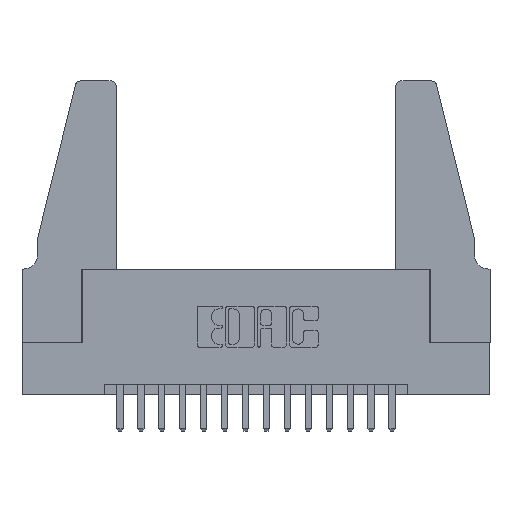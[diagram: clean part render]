
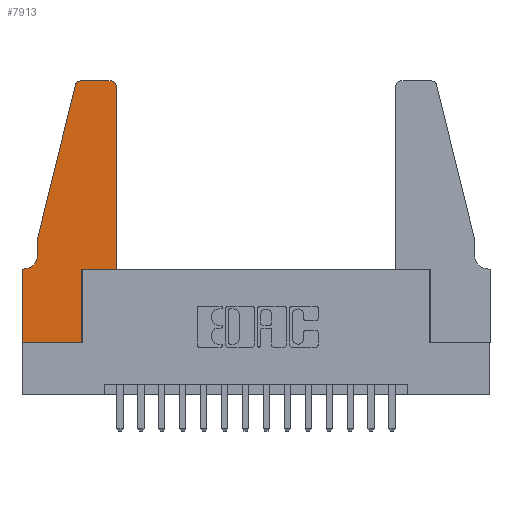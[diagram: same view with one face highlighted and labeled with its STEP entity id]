
A CAD part, top view. The second image highlights one B-rep face of the part: STEP entity #7913.
In plain terms, the highlighted planar face has unit normal (0, 0, 1).
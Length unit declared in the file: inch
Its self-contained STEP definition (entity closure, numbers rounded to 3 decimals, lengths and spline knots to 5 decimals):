
#458 = LINE ( 'NONE', #13785, #7588 ) ;
#483 = ORIENTED_EDGE ( 'NONE', *, *, #13686, .T. ) ;
#556 = CARTESIAN_POINT ( 'NONE',  ( 0., 0.35, 0.37 ) ) ;
#858 = EDGE_CURVE ( 'NONE', #5133, #15432, #12347, .T. ) ;
#1026 = DIRECTION ( 'NONE',  ( -0.239, -0.971, 0. ) ) ;
#1693 = VECTOR ( 'NONE', #9237, 39.37008 ) ;
#1851 = CARTESIAN_POINT ( 'NONE',  ( 0.4505, 1.22, 0.37 ) ) ;
#2402 = CARTESIAN_POINT ( 'NONE',  ( 0.4205, 1.25, 0.37 ) ) ;
#2616 = VECTOR ( 'NONE', #14030, 39.37008 ) ;
#3162 = EDGE_CURVE ( 'NONE', #16909, #5133, #6333, .T. ) ;
#3277 = DIRECTION ( 'NONE',  ( 1., 0., 0. ) ) ;
#3656 = VERTEX_POINT ( 'NONE', #10121 ) ;
#4007 = EDGE_LOOP ( 'NONE', ( #9129, #13714, #14220, #9911, #16022, #4185, #13271, #483, #8920, #12333, #10985, #10590 ) ) ;
#4185 = ORIENTED_EDGE ( 'NONE', *, *, #858, .T. ) ;
#4393 = EDGE_CURVE ( 'NONE', #14015, #13728, #16168, .T. ) ;
#4400 = VERTEX_POINT ( 'NONE', #2402 ) ;
#4958 = CARTESIAN_POINT ( 'NONE',  ( 0.0055, 0.42, 0.37 ) ) ;
#5133 = VERTEX_POINT ( 'NONE', #14228 ) ;
#5149 = CARTESIAN_POINT ( 'NONE',  ( 0.2865, 0., 0.37 ) ) ;
#5242 = LINE ( 'NONE', #13242, #12202 ) ;
#5379 = VECTOR ( 'NONE', #9715, 39.37008 ) ;
#5393 = DIRECTION ( 'NONE',  ( -1., 0., 0. ) ) ;
#5952 = DIRECTION ( 'NONE',  ( 0., 0., 1. ) ) ;
#6082 = CARTESIAN_POINT ( 'NONE',  ( 0.284, 1.25, 0.37 ) ) ;
#6154 = EDGE_CURVE ( 'NONE', #13728, #16909, #13134, .T. ) ;
#6277 = DIRECTION ( 'NONE',  ( -1., 0., 0. ) ) ;
#6333 = CIRCLE ( 'NONE', #15976, 0.07 ) ;
#6568 = CARTESIAN_POINT ( 'NONE',  ( 0.0755, 0.42, 0.37 ) ) ;
#6628 = CARTESIAN_POINT ( 'NONE',  ( 0.0755, 0.5, 0.37 ) ) ;
#6724 = CARTESIAN_POINT ( 'NONE',  ( 0.4505, 0.35, 0.37 ) ) ;
#7111 = DIRECTION ( 'NONE',  ( 0., 0., 1. ) ) ;
#7262 = DIRECTION ( 'NONE',  ( 1., 0., 0. ) ) ;
#7545 = CARTESIAN_POINT ( 'NONE',  ( 0.2865, 0.35, 0.37 ) ) ;
#7588 = VECTOR ( 'NONE', #7262, 39.37008 ) ;
#7666 = VERTEX_POINT ( 'NONE', #6724 ) ;
#7913 = ADVANCED_FACE ( 'NONE', ( #14283 ), #13766, .T. ) ;
#8058 = CIRCLE ( 'NONE', #16839, 0.03 ) ;
#8786 = EDGE_CURVE ( 'NONE', #7666, #14773, #10790, .T. ) ;
#8920 = ORIENTED_EDGE ( 'NONE', *, *, #12133, .T. ) ;
#9095 = AXIS2_PLACEMENT_3D ( 'NONE', #556, #11200, #3277 ) ;
#9129 = ORIENTED_EDGE ( 'NONE', *, *, #14505, .T. ) ;
#9237 = DIRECTION ( 'NONE',  ( 1., 0., 0. ) ) ;
#9715 = DIRECTION ( 'NONE',  ( -1., 0., 0. ) ) ;
#9911 = ORIENTED_EDGE ( 'NONE', *, *, #6154, .T. ) ;
#10121 = CARTESIAN_POINT ( 'NONE',  ( 0., 0., 0.37 ) ) ;
#10391 = VECTOR ( 'NONE', #13897, 39.37008 ) ;
#10497 = EDGE_CURVE ( 'NONE', #15541, #14015, #16720, .T. ) ;
#10590 = ORIENTED_EDGE ( 'NONE', *, *, #16081, .T. ) ;
#10790 = LINE ( 'NONE', #12587, #10391 ) ;
#10819 = VERTEX_POINT ( 'NONE', #16767 ) ;
#10985 = ORIENTED_EDGE ( 'NONE', *, *, #8786, .T. ) ;
#11200 = DIRECTION ( 'NONE',  ( 0., 0., 1. ) ) ;
#11988 = EDGE_CURVE ( 'NONE', #10819, #7666, #458, .T. ) ;
#11992 = VECTOR ( 'NONE', #13680, 39.37008 ) ;
#12087 = VECTOR ( 'NONE', #16584, 39.37008 ) ;
#12133 = EDGE_CURVE ( 'NONE', #13599, #10819, #15098, .T. ) ;
#12202 = VECTOR ( 'NONE', #5393, 39.37008 ) ;
#12333 = ORIENTED_EDGE ( 'NONE', *, *, #11988, .T. ) ;
#12347 = LINE ( 'NONE', #15831, #5379 ) ;
#12398 = LINE ( 'NONE', #16216, #11992 ) ;
#12466 = CARTESIAN_POINT ( 'NONE',  ( 0.25487, 1.22718, 0.37 ) ) ;
#12587 = CARTESIAN_POINT ( 'NONE',  ( 0.4505, 0.35, 0.37 ) ) ;
#12721 = CARTESIAN_POINT ( 'NONE',  ( 0.0755, 0.5, 0.37 ) ) ;
#12773 = VECTOR ( 'NONE', #1026, 39.37008 ) ;
#12838 = AXIS2_PLACEMENT_3D ( 'NONE', #14897, #7111, #16167 ) ;
#13134 = LINE ( 'NONE', #12721, #2616 ) ;
#13170 = CARTESIAN_POINT ( 'NONE',  ( 0., 0., 0.37 ) ) ;
#13242 = CARTESIAN_POINT ( 'NONE',  ( 0.2605, 1.25, 0.37 ) ) ;
#13271 = ORIENTED_EDGE ( 'NONE', *, *, #14752, .T. ) ;
#13599 = VERTEX_POINT ( 'NONE', #5149 ) ;
#13680 = DIRECTION ( 'NONE',  ( 0., -1., 0. ) ) ;
#13686 = EDGE_CURVE ( 'NONE', #3656, #13599, #16426, .T. ) ;
#13714 = ORIENTED_EDGE ( 'NONE', *, *, #10497, .T. ) ;
#13728 = VERTEX_POINT ( 'NONE', #6628 ) ;
#13766 = PLANE ( 'NONE',  #9095 ) ;
#13785 = CARTESIAN_POINT ( 'NONE',  ( 0.4505, 0.35, 0.37 ) ) ;
#13806 = CARTESIAN_POINT ( 'NONE',  ( 0.4205, 1.22, 0.37 ) ) ;
#13897 = DIRECTION ( 'NONE',  ( 0., 1., 0. ) ) ;
#14015 = VERTEX_POINT ( 'NONE', #12466 ) ;
#14030 = DIRECTION ( 'NONE',  ( 0., -1., 0. ) ) ;
#14113 = DIRECTION ( 'NONE',  ( 0., 0., -1. ) ) ;
#14220 = ORIENTED_EDGE ( 'NONE', *, *, #4393, .T. ) ;
#14228 = CARTESIAN_POINT ( 'NONE',  ( 0.0055, 0.35, 0.37 ) ) ;
#14283 = FACE_OUTER_BOUND ( 'NONE', #4007, .T. ) ;
#14505 = EDGE_CURVE ( 'NONE', #4400, #15541, #5242, .T. ) ;
#14752 = EDGE_CURVE ( 'NONE', #15432, #3656, #12398, .T. ) ;
#14773 = VERTEX_POINT ( 'NONE', #1851 ) ;
#14897 = CARTESIAN_POINT ( 'NONE',  ( 0.284, 1.22, 0.37 ) ) ;
#15035 = CARTESIAN_POINT ( 'NONE',  ( 0., 0.35, 0.37 ) ) ;
#15068 = DIRECTION ( 'NONE',  ( 1., 0., 0. ) ) ;
#15098 = LINE ( 'NONE', #7545, #12087 ) ;
#15432 = VERTEX_POINT ( 'NONE', #15035 ) ;
#15541 = VERTEX_POINT ( 'NONE', #6082 ) ;
#15831 = CARTESIAN_POINT ( 'NONE',  ( 0.0755, 0.35, 0.37 ) ) ;
#15976 = AXIS2_PLACEMENT_3D ( 'NONE', #4958, #14113, #6277 ) ;
#16022 = ORIENTED_EDGE ( 'NONE', *, *, #3162, .T. ) ;
#16081 = EDGE_CURVE ( 'NONE', #14773, #4400, #8058, .T. ) ;
#16167 = DIRECTION ( 'NONE',  ( 1., 0., 0. ) ) ;
#16168 = LINE ( 'NONE', #16726, #12773 ) ;
#16216 = CARTESIAN_POINT ( 'NONE',  ( 0., 0., 0.37 ) ) ;
#16426 = LINE ( 'NONE', #13170, #1693 ) ;
#16584 = DIRECTION ( 'NONE',  ( 0., 1., 0. ) ) ;
#16720 = CIRCLE ( 'NONE', #12838, 0.03 ) ;
#16726 = CARTESIAN_POINT ( 'NONE',  ( 0.0755, 0.5, 0.37 ) ) ;
#16767 = CARTESIAN_POINT ( 'NONE',  ( 0.2865, 0.35, 0.37 ) ) ;
#16839 = AXIS2_PLACEMENT_3D ( 'NONE', #13806, #5952, #15068 ) ;
#16909 = VERTEX_POINT ( 'NONE', #6568 ) ;
